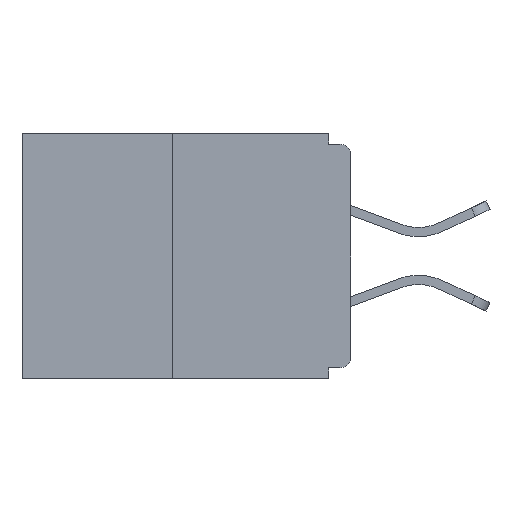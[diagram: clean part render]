
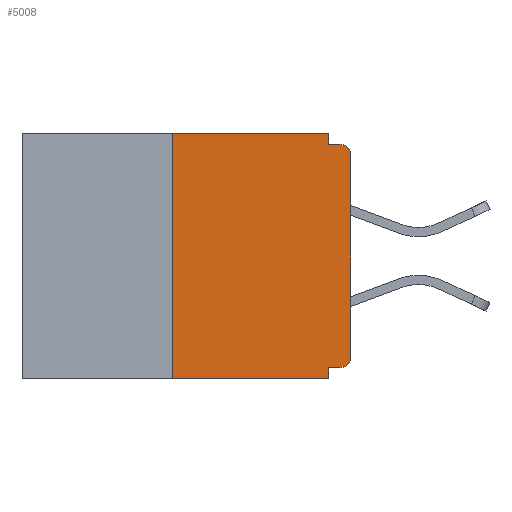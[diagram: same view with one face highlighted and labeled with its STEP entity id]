
A CAD part, left-side view. The second image highlights one B-rep face of the part: STEP entity #5008.
In plain terms, the highlighted planar face has unit normal (-1, 0, 0).
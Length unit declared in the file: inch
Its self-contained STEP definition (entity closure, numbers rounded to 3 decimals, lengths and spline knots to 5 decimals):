
#292 = CARTESIAN_POINT ( 'NONE',  ( 0., 0.015, -0.313 ) ) ;
#325 = DIRECTION ( 'NONE',  ( 0., 1., 0. ) ) ;
#408 = ORIENTED_EDGE ( 'NONE', *, *, #14242, .F. ) ;
#410 = AXIS2_PLACEMENT_3D ( 'NONE', #11110, #12334, #4889 ) ;
#662 = CIRCLE ( 'NONE', #410, 0.015 ) ;
#780 = VERTEX_POINT ( 'NONE', #14327 ) ;
#859 = LINE ( 'NONE', #9296, #11557 ) ;
#995 = CARTESIAN_POINT ( 'NONE',  ( 0., 0., -0.015 ) ) ;
#1035 = CARTESIAN_POINT ( 'NONE',  ( 0., 0.25, -0.343 ) ) ;
#1101 = DIRECTION ( 'NONE',  ( 0., 0., -1. ) ) ;
#1276 = VERTEX_POINT ( 'NONE', #5318 ) ;
#1520 = CARTESIAN_POINT ( 'NONE',  ( 0., 0.015, -0.015 ) ) ;
#1523 = VECTOR ( 'NONE', #3058, 39.37008 ) ;
#1641 = DIRECTION ( 'NONE',  ( 0., 0., -1. ) ) ;
#2000 = VERTEX_POINT ( 'NONE', #9714 ) ;
#2045 = VECTOR ( 'NONE', #7817, 39.37008 ) ;
#2164 = CIRCLE ( 'NONE', #5829, 0.015 ) ;
#2673 = LINE ( 'NONE', #7453, #9712 ) ;
#2718 = ORIENTED_EDGE ( 'NONE', *, *, #12041, .T. ) ;
#2762 = ORIENTED_EDGE ( 'NONE', *, *, #13812, .F. ) ;
#2779 = EDGE_CURVE ( 'NONE', #4510, #15093, #662, .T. ) ;
#2825 = CARTESIAN_POINT ( 'NONE',  ( 0., 0.46, 0. ) ) ;
#3058 = DIRECTION ( 'NONE',  ( 0., 0., 1. ) ) ;
#3081 = CARTESIAN_POINT ( 'NONE',  ( 0., 0., -0.03 ) ) ;
#3927 = ORIENTED_EDGE ( 'NONE', *, *, #2779, .T. ) ;
#4007 = PLANE ( 'NONE',  #13275 ) ;
#4072 = VERTEX_POINT ( 'NONE', #15503 ) ;
#4152 = VERTEX_POINT ( 'NONE', #1035 ) ;
#4280 = ORIENTED_EDGE ( 'NONE', *, *, #11902, .F. ) ;
#4510 = VERTEX_POINT ( 'NONE', #3081 ) ;
#4523 = CARTESIAN_POINT ( 'NONE',  ( 0., 0., -0.313 ) ) ;
#4833 = ORIENTED_EDGE ( 'NONE', *, *, #16015, .T. ) ;
#4889 = DIRECTION ( 'NONE',  ( 0., 0., -1. ) ) ;
#4961 = EDGE_CURVE ( 'NONE', #2000, #9412, #15080, .T. ) ;
#5008 = ADVANCED_FACE ( 'NONE', ( #13527 ), #4007, .F. ) ;
#5067 = CARTESIAN_POINT ( 'NONE',  ( 0., 0.031, 0. ) ) ;
#5091 = LINE ( 'NONE', #14301, #7065 ) ;
#5318 = CARTESIAN_POINT ( 'NONE',  ( 0., 0.031, -0.343 ) ) ;
#5587 = EDGE_CURVE ( 'NONE', #13085, #780, #859, .T. ) ;
#5657 = EDGE_LOOP ( 'NONE', ( #11403, #408, #2718, #2762, #11579, #9591, #4833, #3927, #4280, #8806 ) ) ;
#5829 = AXIS2_PLACEMENT_3D ( 'NONE', #292, #8001, #11457 ) ;
#6447 = LINE ( 'NONE', #995, #9791 ) ;
#6625 = LINE ( 'NONE', #7576, #15986 ) ;
#7065 = VECTOR ( 'NONE', #15668, 39.37008 ) ;
#7364 = CARTESIAN_POINT ( 'NONE',  ( 0., 0.031, -0.343 ) ) ;
#7453 = CARTESIAN_POINT ( 'NONE',  ( 0., 0.031, 0. ) ) ;
#7576 = CARTESIAN_POINT ( 'NONE',  ( 0., 0.46, -0.343 ) ) ;
#7817 = DIRECTION ( 'NONE',  ( 0., -1., 0. ) ) ;
#7918 = DIRECTION ( 'NONE',  ( 1., 0., 0. ) ) ;
#8001 = DIRECTION ( 'NONE',  ( -1., 0., 0. ) ) ;
#8199 = VERTEX_POINT ( 'NONE', #4523 ) ;
#8715 = DIRECTION ( 'NONE',  ( 0., 0., -1. ) ) ;
#8806 = ORIENTED_EDGE ( 'NONE', *, *, #14568, .F. ) ;
#8845 = DIRECTION ( 'NONE',  ( 0., -1., 0. ) ) ;
#8973 = CARTESIAN_POINT ( 'NONE',  ( 0., 0.46, 0. ) ) ;
#9296 = CARTESIAN_POINT ( 'NONE',  ( 0., 0., -0.328 ) ) ;
#9412 = VERTEX_POINT ( 'NONE', #5067 ) ;
#9591 = ORIENTED_EDGE ( 'NONE', *, *, #11703, .T. ) ;
#9712 = VECTOR ( 'NONE', #8715, 39.37008 ) ;
#9714 = CARTESIAN_POINT ( 'NONE',  ( 0., 0.25, 0. ) ) ;
#9791 = VECTOR ( 'NONE', #13393, 39.37008 ) ;
#10112 = VECTOR ( 'NONE', #1101, 39.37008 ) ;
#10179 = CARTESIAN_POINT ( 'NONE',  ( 0., 0.015, -0.328 ) ) ;
#11110 = CARTESIAN_POINT ( 'NONE',  ( 0., 0.015, -0.03 ) ) ;
#11403 = ORIENTED_EDGE ( 'NONE', *, *, #4961, .F. ) ;
#11457 = DIRECTION ( 'NONE',  ( 0., 0., -1. ) ) ;
#11557 = VECTOR ( 'NONE', #325, 39.37008 ) ;
#11579 = ORIENTED_EDGE ( 'NONE', *, *, #5587, .F. ) ;
#11703 = EDGE_CURVE ( 'NONE', #13085, #8199, #2164, .T. ) ;
#11902 = EDGE_CURVE ( 'NONE', #4072, #15093, #6447, .T. ) ;
#12041 = EDGE_CURVE ( 'NONE', #4152, #1276, #6625, .T. ) ;
#12334 = DIRECTION ( 'NONE',  ( -1., 0., 0. ) ) ;
#13037 = CARTESIAN_POINT ( 'NONE',  ( 0., 0.25, 0. ) ) ;
#13085 = VERTEX_POINT ( 'NONE', #10179 ) ;
#13275 = AXIS2_PLACEMENT_3D ( 'NONE', #2825, #7918, #1641 ) ;
#13393 = DIRECTION ( 'NONE',  ( 0., -1., 0. ) ) ;
#13527 = FACE_OUTER_BOUND ( 'NONE', #5657, .T. ) ;
#13812 = EDGE_CURVE ( 'NONE', #780, #1276, #14748, .T. ) ;
#14171 = LINE ( 'NONE', #13037, #1523 ) ;
#14242 = EDGE_CURVE ( 'NONE', #4152, #2000, #14171, .T. ) ;
#14301 = CARTESIAN_POINT ( 'NONE',  ( 0., 0., 0. ) ) ;
#14327 = CARTESIAN_POINT ( 'NONE',  ( 0., 0.031, -0.328 ) ) ;
#14568 = EDGE_CURVE ( 'NONE', #9412, #4072, #2673, .T. ) ;
#14748 = LINE ( 'NONE', #7364, #10112 ) ;
#15080 = LINE ( 'NONE', #8973, #2045 ) ;
#15093 = VERTEX_POINT ( 'NONE', #1520 ) ;
#15503 = CARTESIAN_POINT ( 'NONE',  ( 0., 0.031, -0.015 ) ) ;
#15668 = DIRECTION ( 'NONE',  ( 0., 0., 1. ) ) ;
#15986 = VECTOR ( 'NONE', #8845, 39.37008 ) ;
#16015 = EDGE_CURVE ( 'NONE', #8199, #4510, #5091, .T. ) ;
